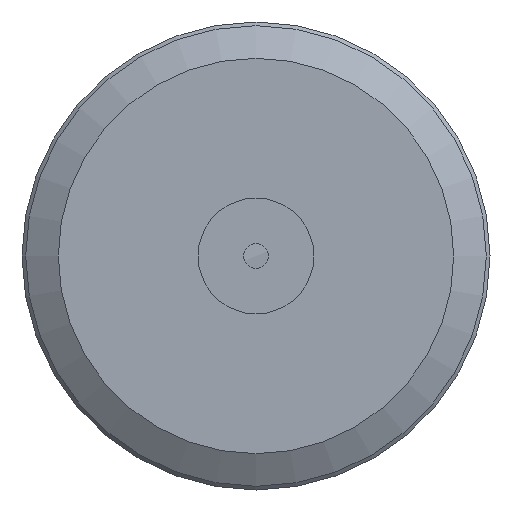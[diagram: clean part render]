
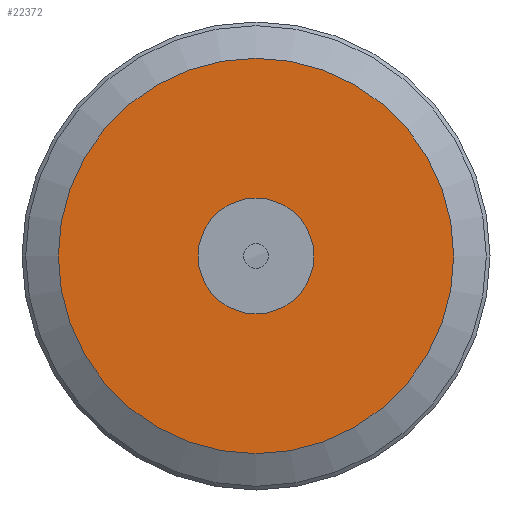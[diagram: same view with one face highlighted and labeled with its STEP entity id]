
A CAD part, front view. The second image highlights one B-rep face of the part: STEP entity #22372.
In plain terms, the highlighted planar face has unit normal (0, -1, 0).
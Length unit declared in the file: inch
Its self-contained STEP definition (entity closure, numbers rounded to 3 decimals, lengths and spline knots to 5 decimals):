
#22041=CARTESIAN_POINT('',(-0.5635,0.,0.0));
#22042=VERTEX_POINT('',#22041);
#22043=CARTESIAN_POINT('',(0.0,0.,0.0));
#22044=DIRECTION('',(0.0,1.0,0.0));
#22045=DIRECTION('',(-1.0,0.0,0.0));
#22046=AXIS2_PLACEMENT_3D('',#22043,#22044,#22045);
#22047=CIRCLE('',#22046,0.5635);
#22048=EDGE_CURVE('',#22042,#22042,#22047,.T.);
#22346=CARTESIAN_POINT('',(-0.165,0.,0.0));
#22347=VERTEX_POINT('',#22346);
#22348=CARTESIAN_POINT('',(0.0,0.,0.0));
#22349=DIRECTION('',(0.0,1.0,0.0));
#22350=DIRECTION('',(-1.0,0.0,0.0));
#22351=AXIS2_PLACEMENT_3D('',#22348,#22349,#22350);
#22352=CIRCLE('',#22351,0.165);
#22353=EDGE_CURVE('',#22347,#22347,#22352,.T.);
#22361=CARTESIAN_POINT('',(-0.36425,0.,0.0));
#22362=DIRECTION('',(0.0,-1.0,0.0));
#22363=DIRECTION('',(0.0,0.0,-1.0));
#22364=AXIS2_PLACEMENT_3D('',#22361,#22362,#22363);
#22365=PLANE('',#22364);
#22366=ORIENTED_EDGE('',*,*,#22048,.F.);
#22367=EDGE_LOOP('',(#22366));
#22368=FACE_OUTER_BOUND('',#22367,.T.);
#22369=ORIENTED_EDGE('',*,*,#22353,.T.);
#22370=EDGE_LOOP('',(#22369));
#22371=FACE_BOUND('',#22370,.T.);
#22372=ADVANCED_FACE('',(#22368,#22371),#22365,.T.);
